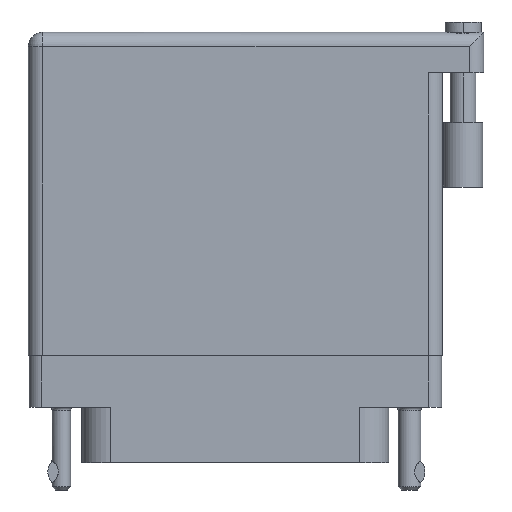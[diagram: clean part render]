
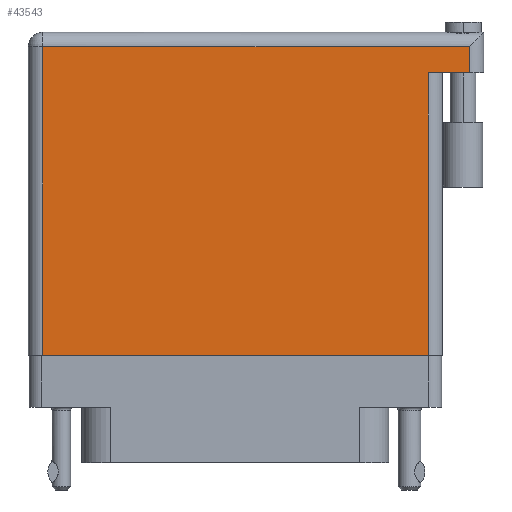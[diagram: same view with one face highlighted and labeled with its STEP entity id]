
A CAD part, front view. The second image highlights one B-rep face of the part: STEP entity #43543.
In plain terms, the highlighted face is planar.
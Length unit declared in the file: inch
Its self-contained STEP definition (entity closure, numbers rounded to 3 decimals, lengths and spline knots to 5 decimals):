
#1650 = VECTOR ( 'NONE', #18719, 39.37008 ) ;
#2579 = ORIENTED_EDGE ( 'NONE', *, *, #30249, .T. ) ;
#3567 = CARTESIAN_POINT ( 'NONE',  ( 1.134, 1.269, 0.4495 ) ) ;
#4286 = CARTESIAN_POINT ( 'NONE',  ( -1.004, 1.466, 0.4495 ) ) ;
#4507 = VECTOR ( 'NONE', #15334, 39.37008 ) ;
#5172 = VERTEX_POINT ( 'NONE', #43831 ) ;
#6792 = EDGE_CURVE ( 'NONE', #30957, #30642, #35366, .T. ) ;
#7074 = VECTOR ( 'NONE', #44565, 39.37008 ) ;
#10221 = VERTEX_POINT ( 'NONE', #14534 ) ;
#10324 = CARTESIAN_POINT ( 'NONE',  ( 1.134, 1.466, 0.4495 ) ) ;
#11342 = LINE ( 'NONE', #27099, #25505 ) ;
#12073 = DIRECTION ( 'NONE',  ( -1., 0., 0. ) ) ;
#14043 = LINE ( 'NONE', #10324, #38898 ) ;
#14534 = CARTESIAN_POINT ( 'NONE',  ( 0.934, -0.1, 0.4495 ) ) ;
#15334 = DIRECTION ( 'NONE',  ( 0., -1., 0. ) ) ;
#15841 = ORIENTED_EDGE ( 'NONE', *, *, #26467, .T. ) ;
#16539 = ORIENTED_EDGE ( 'NONE', *, *, #30908, .T. ) ;
#18185 = CARTESIAN_POINT ( 'NONE',  ( 0.934, 1.269, 0.4495 ) ) ;
#18339 = CARTESIAN_POINT ( 'NONE',  ( 0.934, 1.269, 0.4495 ) ) ;
#18618 = PLANE ( 'NONE',  #26765 ) ;
#18719 = DIRECTION ( 'NONE',  ( 1., 0., 0. ) ) ;
#21166 = VERTEX_POINT ( 'NONE', #44094 ) ;
#22302 = CARTESIAN_POINT ( 'NONE',  ( -0.934, -0.1, 0.4495 ) ) ;
#22490 = ORIENTED_EDGE ( 'NONE', *, *, #6792, .F. ) ;
#23081 = DIRECTION ( 'NONE',  ( -1., 0., 0. ) ) ;
#25505 = VECTOR ( 'NONE', #12073, 39.37008 ) ;
#25751 = LINE ( 'NONE', #18185, #37563 ) ;
#26386 = DIRECTION ( 'NONE',  ( 0., 0., -1. ) ) ;
#26467 = EDGE_CURVE ( 'NONE', #10221, #30642, #25751, .T. ) ;
#26765 = AXIS2_PLACEMENT_3D ( 'NONE', #4286, #26386, #23081 ) ;
#27099 = CARTESIAN_POINT ( 'NONE',  ( -1.004, 1.396, 0.4495 ) ) ;
#28396 = EDGE_LOOP ( 'NONE', ( #16539, #15841, #22490, #2579, #36206, #39035 ) ) ;
#30249 = EDGE_CURVE ( 'NONE', #30957, #5172, #14043, .T. ) ;
#30642 = VERTEX_POINT ( 'NONE', #18339 ) ;
#30908 = EDGE_CURVE ( 'NONE', #44547, #10221, #44196, .T. ) ;
#30957 = VERTEX_POINT ( 'NONE', #3567 ) ;
#33890 = CARTESIAN_POINT ( 'NONE',  ( -1.004, -0.1, 0.4495 ) ) ;
#34442 = FACE_OUTER_BOUND ( 'NONE', #28396, .T. ) ;
#35366 = LINE ( 'NONE', #44412, #7074 ) ;
#36206 = ORIENTED_EDGE ( 'NONE', *, *, #45161, .T. ) ;
#36747 = DIRECTION ( 'NONE',  ( 0., 1., 0. ) ) ;
#37563 = VECTOR ( 'NONE', #48624, 39.37008 ) ;
#38619 = CARTESIAN_POINT ( 'NONE',  ( -0.934, -0.1, 0.4495 ) ) ;
#38898 = VECTOR ( 'NONE', #36747, 39.37008 ) ;
#39035 = ORIENTED_EDGE ( 'NONE', *, *, #43108, .T. ) ;
#43108 = EDGE_CURVE ( 'NONE', #21166, #44547, #43498, .T. ) ;
#43498 = LINE ( 'NONE', #38619, #4507 ) ;
#43543 = ADVANCED_FACE ( 'NONE', ( #34442 ), #18618, .F. ) ;
#43831 = CARTESIAN_POINT ( 'NONE',  ( 1.134, 1.396, 0.4495 ) ) ;
#44094 = CARTESIAN_POINT ( 'NONE',  ( -0.934, 1.396, 0.4495 ) ) ;
#44196 = LINE ( 'NONE', #33890, #1650 ) ;
#44412 = CARTESIAN_POINT ( 'NONE',  ( 1.204, 1.269, 0.4495 ) ) ;
#44547 = VERTEX_POINT ( 'NONE', #22302 ) ;
#44565 = DIRECTION ( 'NONE',  ( -1., 0., 0. ) ) ;
#45161 = EDGE_CURVE ( 'NONE', #5172, #21166, #11342, .T. ) ;
#48624 = DIRECTION ( 'NONE',  ( 0., 1., 0. ) ) ;
